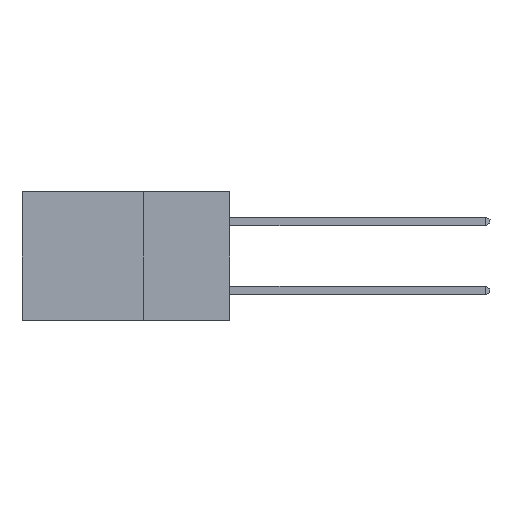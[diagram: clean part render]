
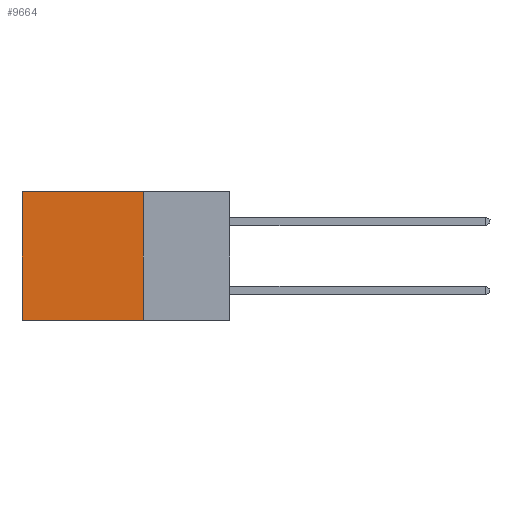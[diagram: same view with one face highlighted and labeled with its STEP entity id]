
A CAD part, left-side view. The second image highlights one B-rep face of the part: STEP entity #9664.
In plain terms, the highlighted planar face has unit normal (-1, 0, 0).
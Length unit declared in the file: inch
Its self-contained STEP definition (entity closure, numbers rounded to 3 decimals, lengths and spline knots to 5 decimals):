
#556 = VERTEX_POINT ( 'NONE', #11570 ) ;
#647 = VERTEX_POINT ( 'NONE', #8343 ) ;
#687 = CARTESIAN_POINT ( 'NONE',  ( 0.2615, 0.25, -0.37 ) ) ;
#701 = EDGE_CURVE ( 'NONE', #10869, #647, #10987, .T. ) ;
#1086 = DIRECTION ( 'NONE',  ( 0., 1., 0. ) ) ;
#1524 = ORIENTED_EDGE ( 'NONE', *, *, #2778, .F. ) ;
#1642 = EDGE_LOOP ( 'NONE', ( #9621, #8883, #1524, #1955 ) ) ;
#1955 = ORIENTED_EDGE ( 'NONE', *, *, #11558, .T. ) ;
#2012 = CARTESIAN_POINT ( 'NONE',  ( 0.2615, 0.25, -0.37 ) ) ;
#2074 = FACE_OUTER_BOUND ( 'NONE', #1642, .T. ) ;
#2778 = EDGE_CURVE ( 'NONE', #556, #4969, #8821, .T. ) ;
#2949 = DIRECTION ( 'NONE',  ( 0., 0., -1. ) ) ;
#3002 = CARTESIAN_POINT ( 'NONE',  ( 0.2615, 0.6, -0.37 ) ) ;
#3086 = DIRECTION ( 'NONE',  ( 0., 0., -1. ) ) ;
#3127 = VECTOR ( 'NONE', #1086, 39.37008 ) ;
#3317 = CARTESIAN_POINT ( 'NONE',  ( 0.2615, 0.25, -0.37 ) ) ;
#3968 = LINE ( 'NONE', #8528, #7364 ) ;
#4729 = DIRECTION ( 'NONE',  ( 0., 1., 0. ) ) ;
#4768 = EDGE_CURVE ( 'NONE', #4969, #647, #7435, .T. ) ;
#4969 = VERTEX_POINT ( 'NONE', #687 ) ;
#6031 = DIRECTION ( 'NONE',  ( 0., 0., -1. ) ) ;
#7364 = VECTOR ( 'NONE', #4729, 39.37008 ) ;
#7435 = LINE ( 'NONE', #2012, #3127 ) ;
#7499 = DIRECTION ( 'NONE',  ( 1., 0., 0. ) ) ;
#8343 = CARTESIAN_POINT ( 'NONE',  ( 0.2615, 0.6, -0.37 ) ) ;
#8528 = CARTESIAN_POINT ( 'NONE',  ( 0.2615, 0.25, 0. ) ) ;
#8821 = LINE ( 'NONE', #3317, #9278 ) ;
#8883 = ORIENTED_EDGE ( 'NONE', *, *, #4768, .F. ) ;
#9196 = AXIS2_PLACEMENT_3D ( 'NONE', #9428, #7499, #3086 ) ;
#9250 = PLANE ( 'NONE',  #9196 ) ;
#9278 = VECTOR ( 'NONE', #6031, 39.37008 ) ;
#9428 = CARTESIAN_POINT ( 'NONE',  ( 0.2615, 0.25, -0.37 ) ) ;
#9579 = VECTOR ( 'NONE', #2949, 39.37008 ) ;
#9621 = ORIENTED_EDGE ( 'NONE', *, *, #701, .T. ) ;
#9664 = ADVANCED_FACE ( 'NONE', ( #2074 ), #9250, .F. ) ;
#10869 = VERTEX_POINT ( 'NONE', #11590 ) ;
#10987 = LINE ( 'NONE', #3002, #9579 ) ;
#11558 = EDGE_CURVE ( 'NONE', #556, #10869, #3968, .T. ) ;
#11570 = CARTESIAN_POINT ( 'NONE',  ( 0.2615, 0.25, 0. ) ) ;
#11590 = CARTESIAN_POINT ( 'NONE',  ( 0.2615, 0.6, 0. ) ) ;
